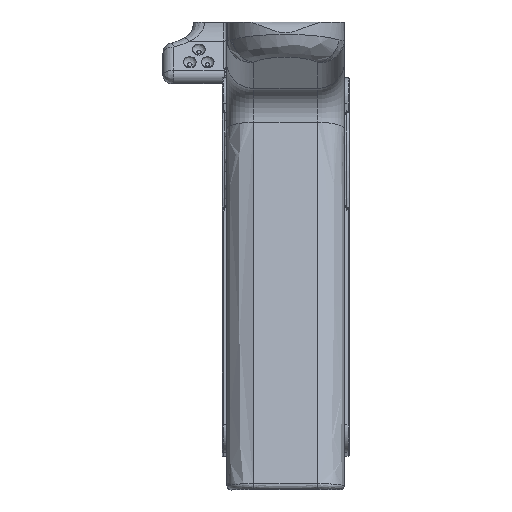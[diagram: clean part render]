
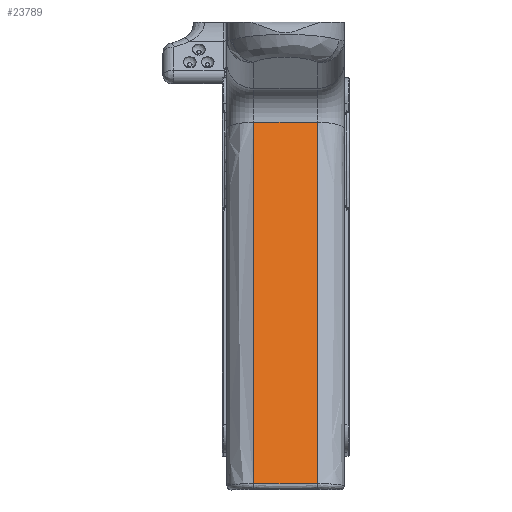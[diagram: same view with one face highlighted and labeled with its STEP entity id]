
A CAD part, front view. The second image highlights one B-rep face of the part: STEP entity #23789.
In plain terms, the highlighted free-form (B-spline) face has degree [5, 1] with [25, 2] control points.
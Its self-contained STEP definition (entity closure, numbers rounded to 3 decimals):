
#913=B_SPLINE_CURVE_WITH_KNOTS('',3,(#31384,#31385,#31386,#31387),
 .UNSPECIFIED.,.F.,.F.,(4,4),(0.,1.495),.UNSPECIFIED.);
#1404=B_SPLINE_CURVE_WITH_KNOTS('',3,(#49537,#49538,#49539,#49540,#49541,
#49542,#49543,#49544,#49545),.UNSPECIFIED.,.F.,.F.,(4,2,1,1,1,4),(-8.931,
-7.453,-6.721,-5.988,-4.523,
-0.128),.UNSPECIFIED.);
#1405=B_SPLINE_CURVE_WITH_KNOTS('',3,(#49598,#49599,#49600,#49601,#49602,
#49603),.UNSPECIFIED.,.F.,.F.,(4,2,4),(-8.803,-1.477,
0.),.UNSPECIFIED.);
#2900=LINE('',#49597,#4501);
#4501=VECTOR('',#28466,6.5);
#6778=FACE_OUTER_BOUND('',#8205,.T.);
#8205=EDGE_LOOP('',(#20261,#20262,#20263,#20264));
#9320=VERTEX_POINT('',#31330);
#9323=VERTEX_POINT('',#31382);
#10937=VERTEX_POINT('',#49480);
#10938=VERTEX_POINT('',#49596);
#11672=EDGE_CURVE('',#9323,#9320,#913,.T.);
#14169=EDGE_CURVE('',#10937,#9323,#1404,.T.);
#14170=EDGE_CURVE('',#10938,#10937,#2900,.T.);
#14171=EDGE_CURVE('',#9320,#10938,#1405,.T.);
#20261=ORIENTED_EDGE('',*,*,#11672,.F.);
#20262=ORIENTED_EDGE('',*,*,#14169,.F.);
#20263=ORIENTED_EDGE('',*,*,#14170,.F.);
#20264=ORIENTED_EDGE('',*,*,#14171,.F.);
#22819=(
BOUNDED_SURFACE()
B_SPLINE_SURFACE(5,1,((#49546,#49547),(#49548,#49549),(#49550,#49551),(#49552,
#49553),(#49554,#49555),(#49556,#49557),(#49558,#49559),(#49560,#49561),
(#49562,#49563),(#49564,#49565),(#49566,#49567),(#49568,#49569),(#49570,
#49571),(#49572,#49573),(#49574,#49575),(#49576,#49577),(#49578,#49579),
(#49580,#49581),(#49582,#49583),(#49584,#49585),(#49586,#49587),(#49588,
#49589),(#49590,#49591),(#49592,#49593),(#49594,#49595)),.UNSPECIFIED.,
 .F.,.F.,.F.)
B_SPLINE_SURFACE_WITH_KNOTS((6,5,1,1,1,1,1,1,1,1,1,5,6),(2,2),(-1.178,
-1.,-0.9,-0.8,-0.7,-0.6,-0.5,-0.4,-0.3,-0.2,-0.1,0.,2.179),(-2.379,
5.132),.UNSPECIFIED.)
GEOMETRIC_REPRESENTATION_ITEM()
RATIONAL_B_SPLINE_SURFACE(((1.,1.),(1.,1.),(1.,1.),(1.,1.),(1.,1.),(1.,
1.),(1.,1.),(1.,1.),(1.,1.),(1.,1.),(1.,1.),(1.,1.),(1.,1.),(1.,1.),(1.,
1.),(1.,1.),(1.,1.),(1.,1.),(1.,1.),(1.,1.),(1.,1.),(1.,1.),(1.,1.),(1.,
1.),(1.,1.)))
REPRESENTATION_ITEM('')
SURFACE()
);
#23789=ADVANCED_FACE('',(#6778),#22819,.F.);
#28466=DIRECTION('',(-1.,0.,0.));
#31330=CARTESIAN_POINT('',(15.925,-90.162,100.53));
#31382=CARTESIAN_POINT('',(0.975,-90.162,100.53));
#31384=CARTESIAN_POINT('Ctrl Pts',(0.975,-90.162,
100.53));
#31385=CARTESIAN_POINT('Ctrl Pts',(5.958,-90.162,100.53));
#31386=CARTESIAN_POINT('Ctrl Pts',(10.942,-90.162,100.53));
#31387=CARTESIAN_POINT('Ctrl Pts',(15.925,-90.162,100.53));
#49480=CARTESIAN_POINT('',(0.975,-66.624,15.913));
#49537=CARTESIAN_POINT('Ctrl Pts',(0.975,-66.624,
15.913));
#49538=CARTESIAN_POINT('Ctrl Pts',(0.975,-67.867,
20.678));
#49539=CARTESIAN_POINT('Ctrl Pts',(0.975,-69.111,
25.444));
#49540=CARTESIAN_POINT('Ctrl Pts',(0.975,-70.968,32.565));
#49541=CARTESIAN_POINT('Ctrl Pts',(0.975,-72.207,37.256));
#49542=CARTESIAN_POINT('Ctrl Pts',(0.975,-74.738,
46.655));
#49543=CARTESIAN_POINT('Ctrl Pts',(0.975,-80.583,67.755));
#49544=CARTESIAN_POINT('Ctrl Pts',(0.975,-86.032,
86.49));
#49545=CARTESIAN_POINT('Ctrl Pts',(0.975,-90.162,
100.53));
#49546=CARTESIAN_POINT('Ctrl Pts',(45.968,-95.649,119.15));
#49547=CARTESIAN_POINT('Ctrl Pts',(-29.15,-95.649,
119.15));
#49548=CARTESIAN_POINT('Ctrl Pts',(45.968,-94.719,115.995));
#49549=CARTESIAN_POINT('Ctrl Pts',(-29.15,-94.719,
115.995));
#49550=CARTESIAN_POINT('Ctrl Pts',(45.968,-93.789,112.841));
#49551=CARTESIAN_POINT('Ctrl Pts',(-29.15,-93.789,112.841));
#49552=CARTESIAN_POINT('Ctrl Pts',(45.968,-92.86,109.686));
#49553=CARTESIAN_POINT('Ctrl Pts',(-29.15,-92.86,
109.686));
#49554=CARTESIAN_POINT('Ctrl Pts',(45.968,-91.93,106.531));
#49555=CARTESIAN_POINT('Ctrl Pts',(-29.15,-91.93,
106.531));
#49556=CARTESIAN_POINT('Ctrl Pts',(45.968,-91.,103.376));
#49557=CARTESIAN_POINT('Ctrl Pts',(-29.15,-91.,
103.376));
#49558=CARTESIAN_POINT('Ctrl Pts',(45.968,-90.477,101.6));
#49559=CARTESIAN_POINT('Ctrl Pts',(-29.15,-90.477,
101.6));
#49560=CARTESIAN_POINT('Ctrl Pts',(45.968,-89.439,98.075));
#49561=CARTESIAN_POINT('Ctrl Pts',(-29.15,-89.439,
98.075));
#49562=CARTESIAN_POINT('Ctrl Pts',(45.968,-87.911,92.865));
#49563=CARTESIAN_POINT('Ctrl Pts',(-29.15,-87.911,
92.865));
#49564=CARTESIAN_POINT('Ctrl Pts',(45.968,-85.928,86.075));
#49565=CARTESIAN_POINT('Ctrl Pts',(-29.15,-85.928,
86.075));
#49566=CARTESIAN_POINT('Ctrl Pts',(45.968,-83.55,77.871));
#49567=CARTESIAN_POINT('Ctrl Pts',(-29.15,-83.55,
77.871));
#49568=CARTESIAN_POINT('Ctrl Pts',(45.968,-81.281,69.978));
#49569=CARTESIAN_POINT('Ctrl Pts',(-29.15,-81.281,
69.978));
#49570=CARTESIAN_POINT('Ctrl Pts',(45.968,-79.134,62.429));
#49571=CARTESIAN_POINT('Ctrl Pts',(-29.15,-79.134,
62.429));
#49572=CARTESIAN_POINT('Ctrl Pts',(45.968,-77.12,55.253));
#49573=CARTESIAN_POINT('Ctrl Pts',(-29.15,-77.12,
55.253));
#49574=CARTESIAN_POINT('Ctrl Pts',(45.968,-75.239,48.457));
#49575=CARTESIAN_POINT('Ctrl Pts',(-29.15,-75.239,
48.457));
#49576=CARTESIAN_POINT('Ctrl Pts',(45.968,-73.485,42.019));
#49577=CARTESIAN_POINT('Ctrl Pts',(-29.15,-73.485,
42.019));
#49578=CARTESIAN_POINT('Ctrl Pts',(45.968,-72.177,37.138));
#49579=CARTESIAN_POINT('Ctrl Pts',(-29.15,-72.177,
37.138));
#49580=CARTESIAN_POINT('Ctrl Pts',(45.968,-71.246,33.618));
#49581=CARTESIAN_POINT('Ctrl Pts',(-29.15,-71.246,33.618));
#49582=CARTESIAN_POINT('Ctrl Pts',(45.968,-70.647,31.334));
#49583=CARTESIAN_POINT('Ctrl Pts',(-29.15,-70.647,
31.334));
#49584=CARTESIAN_POINT('Ctrl Pts',(45.968,-70.353,30.208));
#49585=CARTESIAN_POINT('Ctrl Pts',(-29.15,-70.353,
30.208));
#49586=CARTESIAN_POINT('Ctrl Pts',(45.968,-63.949,5.658));
#49587=CARTESIAN_POINT('Ctrl Pts',(-29.15,-63.949,
5.658));
#49588=CARTESIAN_POINT('Ctrl Pts',(45.968,-57.545,-18.892));
#49589=CARTESIAN_POINT('Ctrl Pts',(-29.15,-57.545,
-18.892));
#49590=CARTESIAN_POINT('Ctrl Pts',(45.968,-51.14,-43.442));
#49591=CARTESIAN_POINT('Ctrl Pts',(-29.15,-51.14,
-43.442));
#49592=CARTESIAN_POINT('Ctrl Pts',(45.968,-44.736,-67.992));
#49593=CARTESIAN_POINT('Ctrl Pts',(-29.15,-44.736,
-67.992));
#49594=CARTESIAN_POINT('Ctrl Pts',(45.968,-38.332,-92.542));
#49595=CARTESIAN_POINT('Ctrl Pts',(-29.15,-38.332,-92.542));
#49596=CARTESIAN_POINT('',(15.925,-66.624,15.913));
#49597=CARTESIAN_POINT('',(22.175,-66.624,15.913));
#49598=CARTESIAN_POINT('Ctrl Pts',(15.925,-90.162,100.53));
#49599=CARTESIAN_POINT('Ctrl Pts',(15.925,-83.279,77.13));
#49600=CARTESIAN_POINT('Ctrl Pts',(15.925,-76.502,53.726));
#49601=CARTESIAN_POINT('Ctrl Pts',(15.925,-69.112,25.456));
#49602=CARTESIAN_POINT('Ctrl Pts',(15.925,-67.867,20.678));
#49603=CARTESIAN_POINT('Ctrl Pts',(15.925,-66.624,15.913));
